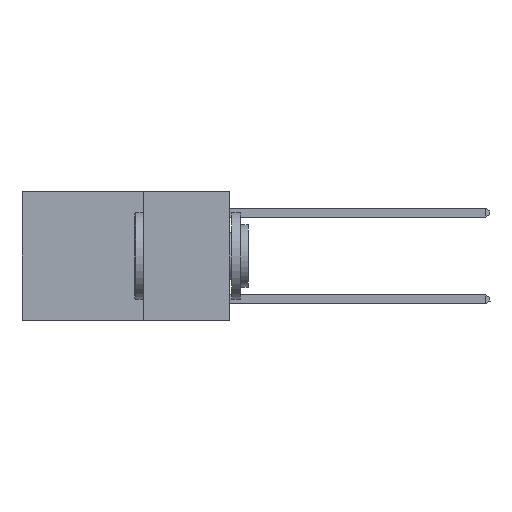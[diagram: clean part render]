
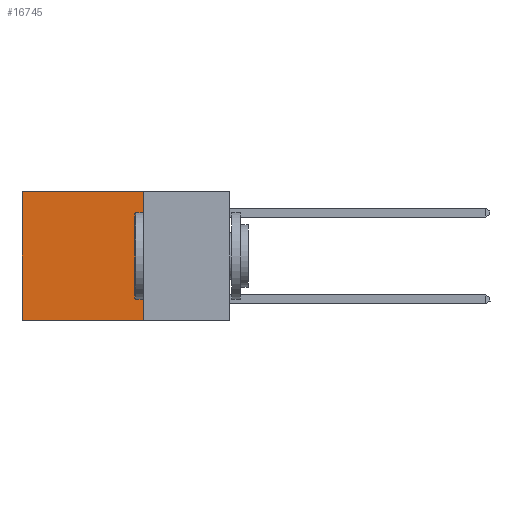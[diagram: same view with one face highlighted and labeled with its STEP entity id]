
A CAD part, left-side view. The second image highlights one B-rep face of the part: STEP entity #16745.
In plain terms, the highlighted planar face has unit normal (-1, 0, 0).
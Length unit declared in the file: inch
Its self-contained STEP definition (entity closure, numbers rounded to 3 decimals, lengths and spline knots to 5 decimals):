
#11 = EDGE_LOOP ( 'NONE', ( #13031, #13049, #13122, #13212 ) ) ;
#1138 = AXIS2_PLACEMENT_3D ( 'NONE', #8252, #3862, #14243 ) ;
#1259 = CARTESIAN_POINT ( 'NONE',  ( 0.2625, 0.25, 0. ) ) ;
#2117 = VERTEX_POINT ( 'NONE', #18117 ) ;
#2728 = LINE ( 'NONE', #16570, #10088 ) ;
#2922 = VECTOR ( 'NONE', #6218, 39.37008 ) ;
#3832 = VERTEX_POINT ( 'NONE', #12766 ) ;
#3862 = DIRECTION ( 'NONE',  ( 1., 0., 0. ) ) ;
#4746 = CARTESIAN_POINT ( 'NONE',  ( 0.2625, 0.6, 0. ) ) ;
#5678 = VECTOR ( 'NONE', #7065, 39.37008 ) ;
#5951 = VERTEX_POINT ( 'NONE', #17544 ) ;
#6218 = DIRECTION ( 'NONE',  ( 0., 0., -1. ) ) ;
#7065 = DIRECTION ( 'NONE',  ( 0., 1., 0. ) ) ;
#7077 = EDGE_CURVE ( 'NONE', #2117, #5951, #11238, .T. ) ;
#8124 = VERTEX_POINT ( 'NONE', #17041 ) ;
#8252 = CARTESIAN_POINT ( 'NONE',  ( 0.2625, 0.25, 0. ) ) ;
#9617 = LINE ( 'NONE', #15999, #5678 ) ;
#9984 = EDGE_CURVE ( 'NONE', #8124, #3832, #17380, .T. ) ;
#10088 = VECTOR ( 'NONE', #11969, 39.37008 ) ;
#11235 = PLANE ( 'NONE',  #1138 ) ;
#11238 = LINE ( 'NONE', #4746, #2922 ) ;
#11623 = DIRECTION ( 'NONE',  ( 0., 0., -1. ) ) ;
#11969 = DIRECTION ( 'NONE',  ( 0., 1., 0. ) ) ;
#12461 = EDGE_CURVE ( 'NONE', #3832, #5951, #9617, .T. ) ;
#12766 = CARTESIAN_POINT ( 'NONE',  ( 0.2625, 0.25, -0.37 ) ) ;
#13031 = ORIENTED_EDGE ( 'NONE', *, *, #7077, .T. ) ;
#13049 = ORIENTED_EDGE ( 'NONE', *, *, #12461, .F. ) ;
#13122 = ORIENTED_EDGE ( 'NONE', *, *, #9984, .F. ) ;
#13212 = ORIENTED_EDGE ( 'NONE', *, *, #16273, .T. ) ;
#13311 = VECTOR ( 'NONE', #11623, 39.37008 ) ;
#14050 = FACE_OUTER_BOUND ( 'NONE', #11, .T. ) ;
#14243 = DIRECTION ( 'NONE',  ( 0., 0., -1. ) ) ;
#15999 = CARTESIAN_POINT ( 'NONE',  ( 0.2625, 0.25, -0.37 ) ) ;
#16273 = EDGE_CURVE ( 'NONE', #8124, #2117, #2728, .T. ) ;
#16570 = CARTESIAN_POINT ( 'NONE',  ( 0.2625, 0.25, 0. ) ) ;
#16745 = ADVANCED_FACE ( 'NONE', ( #14050 ), #11235, .F. ) ;
#17041 = CARTESIAN_POINT ( 'NONE',  ( 0.2625, 0.25, 0. ) ) ;
#17380 = LINE ( 'NONE', #1259, #13311 ) ;
#17544 = CARTESIAN_POINT ( 'NONE',  ( 0.2625, 0.6, -0.37 ) ) ;
#18117 = CARTESIAN_POINT ( 'NONE',  ( 0.2625, 0.6, 0. ) ) ;
